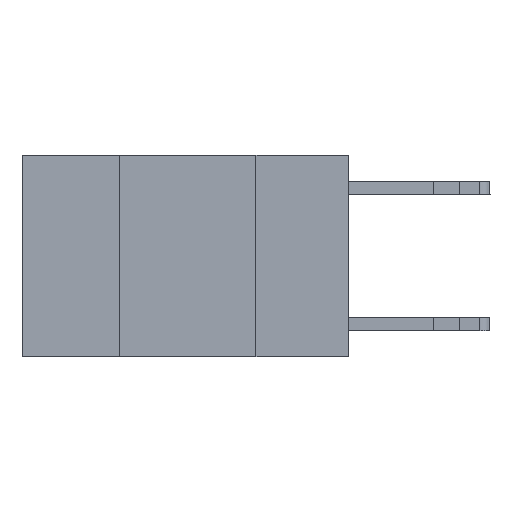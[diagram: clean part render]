
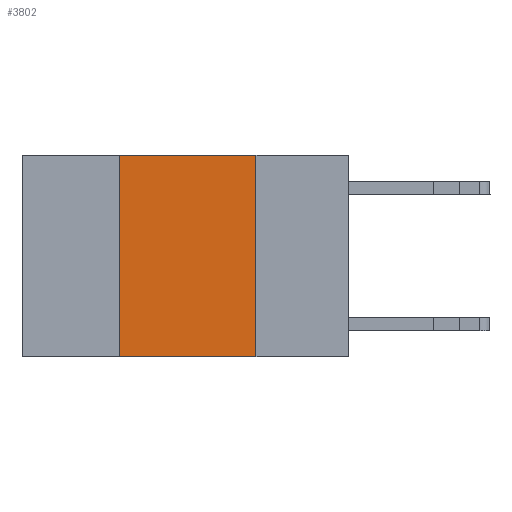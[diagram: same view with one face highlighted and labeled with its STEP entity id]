
A CAD part, left-side view. The second image highlights one B-rep face of the part: STEP entity #3802.
In plain terms, the highlighted planar face has unit normal (-1, 0, 0).
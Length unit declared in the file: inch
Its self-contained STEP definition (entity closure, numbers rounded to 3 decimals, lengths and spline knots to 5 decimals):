
#254 = CARTESIAN_POINT ( 'NONE',  ( 0., 0.6, -0.37 ) ) ;
#543 = VERTEX_POINT ( 'NONE', #3168 ) ;
#895 = CARTESIAN_POINT ( 'NONE',  ( 0., 0.17, -0.37 ) ) ;
#1186 = VECTOR ( 'NONE', #6022, 39.37008 ) ;
#1380 = VERTEX_POINT ( 'NONE', #895 ) ;
#2087 = VERTEX_POINT ( 'NONE', #3843 ) ;
#3122 = VECTOR ( 'NONE', #7326, 39.37008 ) ;
#3168 = CARTESIAN_POINT ( 'NONE',  ( 0., 0.17, 0. ) ) ;
#3618 = LINE ( 'NONE', #5474, #6532 ) ;
#3802 = ADVANCED_FACE ( 'NONE', ( #16877 ), #13235, .F. ) ;
#3843 = CARTESIAN_POINT ( 'NONE',  ( 0., 0.42, -0.37 ) ) ;
#4316 = CARTESIAN_POINT ( 'NONE',  ( 0., 0.6, 0. ) ) ;
#4775 = CARTESIAN_POINT ( 'NONE',  ( 0., 0.6, 0. ) ) ;
#4848 = EDGE_CURVE ( 'NONE', #543, #1380, #3618, .T. ) ;
#5009 = ORIENTED_EDGE ( 'NONE', *, *, #10228, .F. ) ;
#5474 = CARTESIAN_POINT ( 'NONE',  ( 0., 0.17, 0. ) ) ;
#5952 = VERTEX_POINT ( 'NONE', #10592 ) ;
#6022 = DIRECTION ( 'NONE',  ( 0., -1., 0. ) ) ;
#6532 = VECTOR ( 'NONE', #13986, 39.37008 ) ;
#7326 = DIRECTION ( 'NONE',  ( 0., 0., 1. ) ) ;
#7658 = DIRECTION ( 'NONE',  ( 1., 0., 0. ) ) ;
#10019 = AXIS2_PLACEMENT_3D ( 'NONE', #4775, #7658, #17463 ) ;
#10228 = EDGE_CURVE ( 'NONE', #5952, #543, #16729, .T. ) ;
#10592 = CARTESIAN_POINT ( 'NONE',  ( 0., 0.42, 0. ) ) ;
#10684 = LINE ( 'NONE', #15737, #3122 ) ;
#12083 = LINE ( 'NONE', #254, #1186 ) ;
#12840 = EDGE_CURVE ( 'NONE', #2087, #5952, #10684, .T. ) ;
#13235 = PLANE ( 'NONE',  #10019 ) ;
#13559 = EDGE_CURVE ( 'NONE', #2087, #1380, #12083, .T. ) ;
#13986 = DIRECTION ( 'NONE',  ( 0., 0., -1. ) ) ;
#15429 = VECTOR ( 'NONE', #17019, 39.37008 ) ;
#15737 = CARTESIAN_POINT ( 'NONE',  ( 0., 0.42, 0. ) ) ;
#15844 = ORIENTED_EDGE ( 'NONE', *, *, #4848, .F. ) ;
#15935 = EDGE_LOOP ( 'NONE', ( #15844, #5009, #16282, #16713 ) ) ;
#16282 = ORIENTED_EDGE ( 'NONE', *, *, #12840, .F. ) ;
#16713 = ORIENTED_EDGE ( 'NONE', *, *, #13559, .T. ) ;
#16729 = LINE ( 'NONE', #4316, #15429 ) ;
#16877 = FACE_OUTER_BOUND ( 'NONE', #15935, .T. ) ;
#17019 = DIRECTION ( 'NONE',  ( 0., -1., 0. ) ) ;
#17463 = DIRECTION ( 'NONE',  ( 0., 0., -1. ) ) ;
